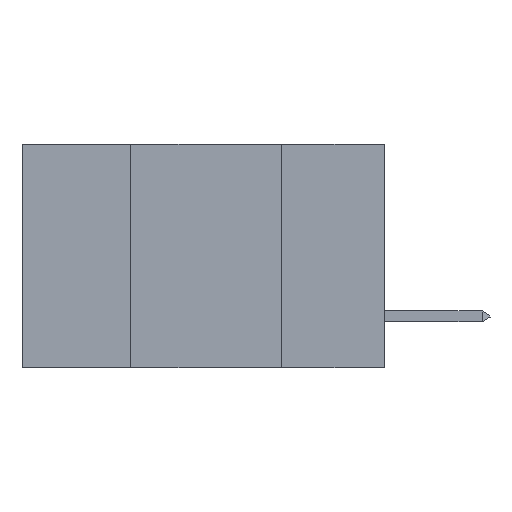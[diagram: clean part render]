
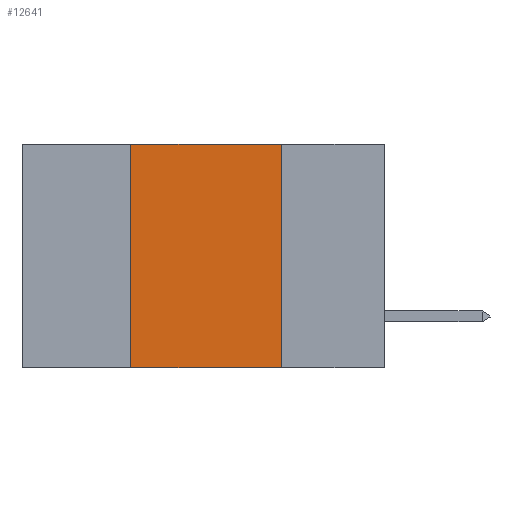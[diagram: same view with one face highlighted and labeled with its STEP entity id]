
A CAD part, left-side view. The second image highlights one B-rep face of the part: STEP entity #12641.
In plain terms, the highlighted planar face has unit normal (-1, 0, 0).
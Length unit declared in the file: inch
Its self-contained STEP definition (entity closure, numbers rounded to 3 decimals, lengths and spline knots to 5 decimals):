
#126 = LINE ( 'NONE', #9324, #12175 ) ;
#591 = DIRECTION ( 'NONE',  ( 0., -1., 0. ) ) ;
#2353 = DIRECTION ( 'NONE',  ( 0., -1., 0. ) ) ;
#2548 = DIRECTION ( 'NONE',  ( 0., 0., -1. ) ) ;
#3428 = PLANE ( 'NONE',  #5832 ) ;
#3659 = VERTEX_POINT ( 'NONE', #14993 ) ;
#3781 = CARTESIAN_POINT ( 'NONE',  ( 0., 0.42, -0.37 ) ) ;
#4384 = VERTEX_POINT ( 'NONE', #3781 ) ;
#5117 = CARTESIAN_POINT ( 'NONE',  ( 0., 0.6, -0.37 ) ) ;
#5298 = EDGE_CURVE ( 'NONE', #3659, #13214, #5340, .T. ) ;
#5340 = LINE ( 'NONE', #5886, #11548 ) ;
#5629 = LINE ( 'NONE', #5117, #13876 ) ;
#5712 = DIRECTION ( 'NONE',  ( 0., 0., 1. ) ) ;
#5832 = AXIS2_PLACEMENT_3D ( 'NONE', #9269, #7180, #2548 ) ;
#5886 = CARTESIAN_POINT ( 'NONE',  ( 0., 0.17, 0. ) ) ;
#6715 = EDGE_CURVE ( 'NONE', #4384, #13508, #14183, .T. ) ;
#7180 = DIRECTION ( 'NONE',  ( 1., 0., 0. ) ) ;
#7944 = ORIENTED_EDGE ( 'NONE', *, *, #13909, .T. ) ;
#9269 = CARTESIAN_POINT ( 'NONE',  ( 0., 0.6, 0. ) ) ;
#9324 = CARTESIAN_POINT ( 'NONE',  ( 0., 0.6, 0. ) ) ;
#9347 = DIRECTION ( 'NONE',  ( 0., 0., -1. ) ) ;
#9382 = FACE_OUTER_BOUND ( 'NONE', #12007, .T. ) ;
#10023 = ORIENTED_EDGE ( 'NONE', *, *, #5298, .F. ) ;
#11292 = EDGE_CURVE ( 'NONE', #13508, #3659, #126, .T. ) ;
#11548 = VECTOR ( 'NONE', #9347, 39.37008 ) ;
#11568 = CARTESIAN_POINT ( 'NONE',  ( 0., 0.42, 0. ) ) ;
#12007 = EDGE_LOOP ( 'NONE', ( #10023, #14081, #13519, #7944 ) ) ;
#12175 = VECTOR ( 'NONE', #2353, 39.37008 ) ;
#12641 = ADVANCED_FACE ( 'NONE', ( #9382 ), #3428, .F. ) ;
#12693 = VECTOR ( 'NONE', #5712, 39.37008 ) ;
#13214 = VERTEX_POINT ( 'NONE', #15006 ) ;
#13508 = VERTEX_POINT ( 'NONE', #13763 ) ;
#13519 = ORIENTED_EDGE ( 'NONE', *, *, #6715, .F. ) ;
#13763 = CARTESIAN_POINT ( 'NONE',  ( 0., 0.42, 0. ) ) ;
#13876 = VECTOR ( 'NONE', #591, 39.37008 ) ;
#13909 = EDGE_CURVE ( 'NONE', #4384, #13214, #5629, .T. ) ;
#14081 = ORIENTED_EDGE ( 'NONE', *, *, #11292, .F. ) ;
#14183 = LINE ( 'NONE', #11568, #12693 ) ;
#14993 = CARTESIAN_POINT ( 'NONE',  ( 0., 0.17, 0. ) ) ;
#15006 = CARTESIAN_POINT ( 'NONE',  ( 0., 0.17, -0.37 ) ) ;
